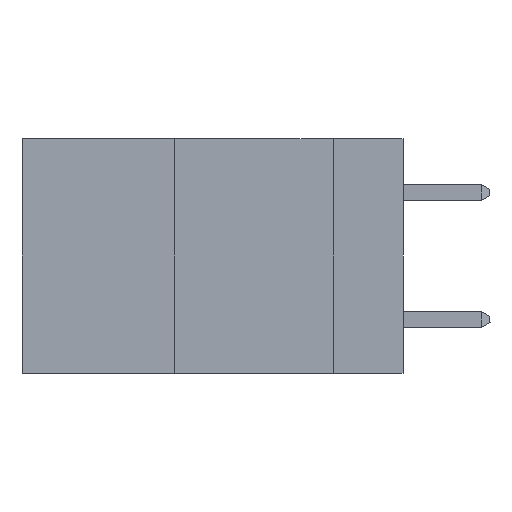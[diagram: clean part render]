
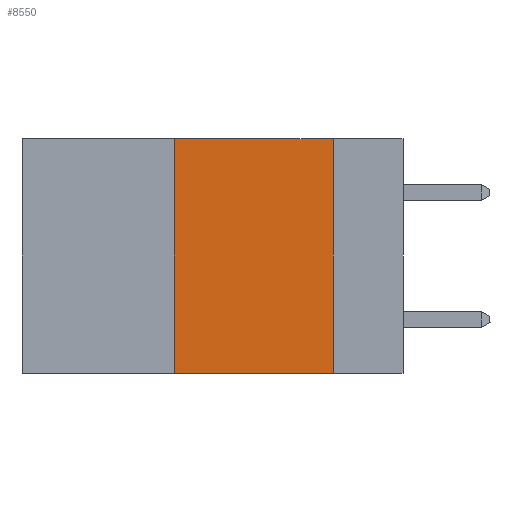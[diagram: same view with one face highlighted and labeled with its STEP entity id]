
A CAD part, left-side view. The second image highlights one B-rep face of the part: STEP entity #8550.
In plain terms, the highlighted planar face has unit normal (-1, 0, 0).
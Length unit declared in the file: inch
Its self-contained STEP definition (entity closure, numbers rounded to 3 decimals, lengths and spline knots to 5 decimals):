
#1053 = DIRECTION ( 'NONE',  ( 0., 0., -1. ) ) ;
#2131 = VERTEX_POINT ( 'NONE', #41288 ) ;
#3208 = EDGE_CURVE ( 'NONE', #31995, #2131, #31489, .T. ) ;
#4184 = ORIENTED_EDGE ( 'NONE', *, *, #3208, .F. ) ;
#5373 = EDGE_CURVE ( 'NONE', #21363, #2131, #19849, .T. ) ;
#8550 = ADVANCED_FACE ( 'NONE', ( #35565 ), #16740, .F. ) ;
#9243 = EDGE_CURVE ( 'NONE', #21363, #28110, #34972, .T. ) ;
#9822 = CARTESIAN_POINT ( 'NONE',  ( 0., 0.36, 0. ) ) ;
#11241 = DIRECTION ( 'NONE',  ( 0., 0., -1. ) ) ;
#14649 = DIRECTION ( 'NONE',  ( 1., 0., 0. ) ) ;
#16136 = CARTESIAN_POINT ( 'NONE',  ( 0., 0.6, -0.37 ) ) ;
#16740 = PLANE ( 'NONE',  #36617 ) ;
#17763 = CARTESIAN_POINT ( 'NONE',  ( 0., 0.6, 0. ) ) ;
#19511 = CARTESIAN_POINT ( 'NONE',  ( 0., 0.6, 0. ) ) ;
#19849 = LINE ( 'NONE', #16136, #27880 ) ;
#21363 = VERTEX_POINT ( 'NONE', #37426 ) ;
#24762 = VECTOR ( 'NONE', #39653, 39.37008 ) ;
#25861 = ORIENTED_EDGE ( 'NONE', *, *, #9243, .F. ) ;
#26988 = ORIENTED_EDGE ( 'NONE', *, *, #33891, .F. ) ;
#27880 = VECTOR ( 'NONE', #36437, 39.37008 ) ;
#28110 = VERTEX_POINT ( 'NONE', #38567 ) ;
#28540 = CARTESIAN_POINT ( 'NONE',  ( 0., 0.11, 0. ) ) ;
#29113 = VECTOR ( 'NONE', #40481, 39.37008 ) ;
#30405 = VECTOR ( 'NONE', #1053, 39.37008 ) ;
#31489 = LINE ( 'NONE', #28540, #30405 ) ;
#31995 = VERTEX_POINT ( 'NONE', #33532 ) ;
#33532 = CARTESIAN_POINT ( 'NONE',  ( 0., 0.11, 0. ) ) ;
#33891 = EDGE_CURVE ( 'NONE', #28110, #31995, #42315, .T. ) ;
#34972 = LINE ( 'NONE', #9822, #29113 ) ;
#35565 = FACE_OUTER_BOUND ( 'NONE', #43396, .T. ) ;
#36437 = DIRECTION ( 'NONE',  ( 0., -1., 0. ) ) ;
#36617 = AXIS2_PLACEMENT_3D ( 'NONE', #17763, #14649, #11241 ) ;
#37426 = CARTESIAN_POINT ( 'NONE',  ( 0., 0.36, -0.37 ) ) ;
#38567 = CARTESIAN_POINT ( 'NONE',  ( 0., 0.36, 0. ) ) ;
#39653 = DIRECTION ( 'NONE',  ( 0., -1., 0. ) ) ;
#40481 = DIRECTION ( 'NONE',  ( 0., 0., 1. ) ) ;
#41288 = CARTESIAN_POINT ( 'NONE',  ( 0., 0.11, -0.37 ) ) ;
#42315 = LINE ( 'NONE', #19511, #24762 ) ;
#43353 = ORIENTED_EDGE ( 'NONE', *, *, #5373, .T. ) ;
#43396 = EDGE_LOOP ( 'NONE', ( #4184, #26988, #25861, #43353 ) ) ;
